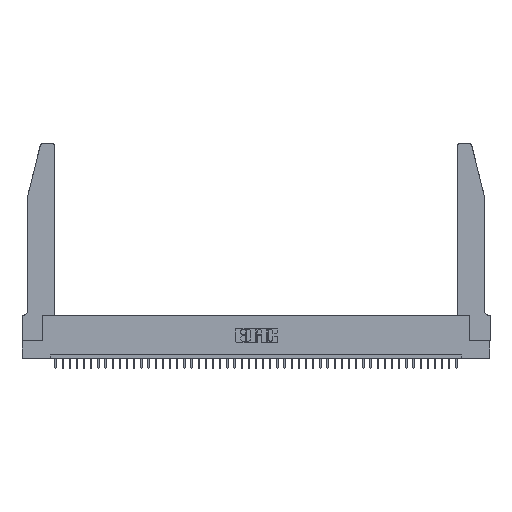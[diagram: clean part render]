
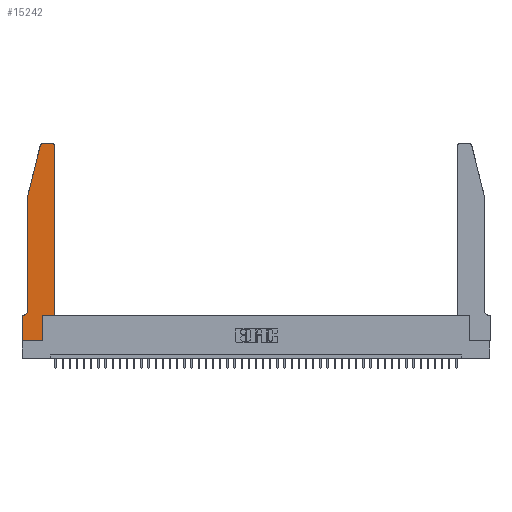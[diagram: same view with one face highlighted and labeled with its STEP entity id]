
A CAD part, top view. The second image highlights one B-rep face of the part: STEP entity #15242.
In plain terms, the highlighted planar face has unit normal (0, 0, 1).
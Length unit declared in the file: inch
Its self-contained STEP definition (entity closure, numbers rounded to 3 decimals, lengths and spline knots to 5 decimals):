
#481 = CARTESIAN_POINT ( 'NONE',  ( 0.25487, 2.72718, 0.37 ) ) ;
#940 = CIRCLE ( 'NONE', #44548, 0.07 ) ;
#1008 = CARTESIAN_POINT ( 'NONE',  ( 0.284, 2.75, 0.37 ) ) ;
#1127 = EDGE_CURVE ( 'NONE', #18805, #17591, #18720, .T. ) ;
#1324 = LINE ( 'NONE', #43206, #7119 ) ;
#1342 = EDGE_CURVE ( 'NONE', #5305, #18805, #2103, .T. ) ;
#2103 = CIRCLE ( 'NONE', #27911, 0.03 ) ;
#2881 = EDGE_CURVE ( 'NONE', #17591, #26068, #1324, .T. ) ;
#3198 = EDGE_CURVE ( 'NONE', #40577, #6330, #34597, .T. ) ;
#3223 = CARTESIAN_POINT ( 'NONE',  ( 0.2865, 0.35, 0.37 ) ) ;
#4160 = CARTESIAN_POINT ( 'NONE',  ( 0.4205, 2.75, 0.37 ) ) ;
#4233 = ORIENTED_EDGE ( 'NONE', *, *, #3198, .T. ) ;
#5054 = DIRECTION ( 'NONE',  ( -1., 0., 0. ) ) ;
#5305 = VERTEX_POINT ( 'NONE', #1008 ) ;
#6330 = VERTEX_POINT ( 'NONE', #33728 ) ;
#6615 = EDGE_CURVE ( 'NONE', #6330, #26174, #14759, .T. ) ;
#6768 = VECTOR ( 'NONE', #5054, 39.37008 ) ;
#7119 = VECTOR ( 'NONE', #15648, 39.37008 ) ;
#7630 = VERTEX_POINT ( 'NONE', #42210 ) ;
#9138 = DIRECTION ( 'NONE',  ( 1., 0., 0. ) ) ;
#9432 = VECTOR ( 'NONE', #25645, 39.37008 ) ;
#9655 = CARTESIAN_POINT ( 'NONE',  ( 0., 0., 0.37 ) ) ;
#10636 = ORIENTED_EDGE ( 'NONE', *, *, #41567, .T. ) ;
#11251 = ORIENTED_EDGE ( 'NONE', *, *, #2881, .T. ) ;
#11930 = DIRECTION ( 'NONE',  ( 0., 0., 1. ) ) ;
#12247 = CARTESIAN_POINT ( 'NONE',  ( 0.0755, 2., 0.37 ) ) ;
#12409 = DIRECTION ( 'NONE',  ( -1., 0., 0. ) ) ;
#12894 = DIRECTION ( 'NONE',  ( 1., 0., 0. ) ) ;
#14079 = CARTESIAN_POINT ( 'NONE',  ( 0., 0.35, 0.37 ) ) ;
#14759 = CIRCLE ( 'NONE', #40643, 0.03 ) ;
#15242 = ADVANCED_FACE ( 'NONE', ( #29955 ), #44088, .T. ) ;
#15648 = DIRECTION ( 'NONE',  ( 0., -1., 0. ) ) ;
#17333 = LINE ( 'NONE', #31433, #22160 ) ;
#17591 = VERTEX_POINT ( 'NONE', #12247 ) ;
#17934 = CARTESIAN_POINT ( 'NONE',  ( 0.4505, 0.35, 0.37 ) ) ;
#18720 = LINE ( 'NONE', #42195, #9432 ) ;
#18805 = VERTEX_POINT ( 'NONE', #481 ) ;
#18978 = CARTESIAN_POINT ( 'NONE',  ( 0.0055, 0.42, 0.37 ) ) ;
#19417 = ORIENTED_EDGE ( 'NONE', *, *, #25958, .T. ) ;
#19795 = VECTOR ( 'NONE', #28095, 39.37008 ) ;
#20864 = EDGE_CURVE ( 'NONE', #36734, #40577, #42946, .T. ) ;
#21230 = CARTESIAN_POINT ( 'NONE',  ( 0., 0., 0.37 ) ) ;
#21503 = ORIENTED_EDGE ( 'NONE', *, *, #20864, .T. ) ;
#22126 = DIRECTION ( 'NONE',  ( 1., 0., 0. ) ) ;
#22160 = VECTOR ( 'NONE', #38630, 39.37008 ) ;
#22268 = EDGE_CURVE ( 'NONE', #38720, #7630, #30485, .T. ) ;
#23160 = EDGE_LOOP ( 'NONE', ( #39592, #43818, #37624, #11251, #27389, #37796, #19417, #27024, #10636, #21503, #4233, #41970 ) ) ;
#23168 = CARTESIAN_POINT ( 'NONE',  ( 0., 0., 0.37 ) ) ;
#23807 = EDGE_CURVE ( 'NONE', #26174, #5305, #40235, .T. ) ;
#24648 = EDGE_CURVE ( 'NONE', #26068, #25562, #940, .T. ) ;
#25562 = VERTEX_POINT ( 'NONE', #34333 ) ;
#25645 = DIRECTION ( 'NONE',  ( -0.239, -0.971, 0. ) ) ;
#25958 = EDGE_CURVE ( 'NONE', #28944, #38720, #41449, .T. ) ;
#26068 = VERTEX_POINT ( 'NONE', #34950 ) ;
#26073 = DIRECTION ( 'NONE',  ( 0., 0., 1. ) ) ;
#26174 = VERTEX_POINT ( 'NONE', #4160 ) ;
#26617 = DIRECTION ( 'NONE',  ( 0., 0., -1. ) ) ;
#27024 = ORIENTED_EDGE ( 'NONE', *, *, #22268, .T. ) ;
#27389 = ORIENTED_EDGE ( 'NONE', *, *, #24648, .T. ) ;
#27911 = AXIS2_PLACEMENT_3D ( 'NONE', #28146, #38590, #45326 ) ;
#28095 = DIRECTION ( 'NONE',  ( 0., 1., 0. ) ) ;
#28146 = CARTESIAN_POINT ( 'NONE',  ( 0.284, 2.72, 0.37 ) ) ;
#28944 = VERTEX_POINT ( 'NONE', #14079 ) ;
#29955 = FACE_OUTER_BOUND ( 'NONE', #23160, .T. ) ;
#30485 = LINE ( 'NONE', #9655, #32506 ) ;
#31433 = CARTESIAN_POINT ( 'NONE',  ( 0.2865, 0.35, 0.37 ) ) ;
#32506 = VECTOR ( 'NONE', #12894, 39.37008 ) ;
#33234 = CARTESIAN_POINT ( 'NONE',  ( 0.0755, 0.35, 0.37 ) ) ;
#33728 = CARTESIAN_POINT ( 'NONE',  ( 0.4505, 2.72, 0.37 ) ) ;
#33906 = CARTESIAN_POINT ( 'NONE',  ( 0.4505, 0.35, 0.37 ) ) ;
#34333 = CARTESIAN_POINT ( 'NONE',  ( 0.0055, 0.35, 0.37 ) ) ;
#34597 = LINE ( 'NONE', #17934, #19795 ) ;
#34950 = CARTESIAN_POINT ( 'NONE',  ( 0.0755, 0.42, 0.37 ) ) ;
#35726 = VECTOR ( 'NONE', #37498, 39.37008 ) ;
#35764 = CARTESIAN_POINT ( 'NONE',  ( 0.4505, 0.35, 0.37 ) ) ;
#36696 = CARTESIAN_POINT ( 'NONE',  ( 0.4205, 2.72, 0.37 ) ) ;
#36723 = CARTESIAN_POINT ( 'NONE',  ( 0.2605, 2.75, 0.37 ) ) ;
#36734 = VERTEX_POINT ( 'NONE', #3223 ) ;
#37009 = EDGE_CURVE ( 'NONE', #25562, #28944, #44360, .T. ) ;
#37498 = DIRECTION ( 'NONE',  ( 0., -1., 0. ) ) ;
#37624 = ORIENTED_EDGE ( 'NONE', *, *, #1127, .T. ) ;
#37796 = ORIENTED_EDGE ( 'NONE', *, *, #37009, .T. ) ;
#38590 = DIRECTION ( 'NONE',  ( 0., 0., 1. ) ) ;
#38630 = DIRECTION ( 'NONE',  ( 0., 1., 0. ) ) ;
#38720 = VERTEX_POINT ( 'NONE', #21230 ) ;
#39592 = ORIENTED_EDGE ( 'NONE', *, *, #23807, .T. ) ;
#39718 = AXIS2_PLACEMENT_3D ( 'NONE', #40851, #11930, #9138 ) ;
#40235 = LINE ( 'NONE', #36723, #6768 ) ;
#40577 = VERTEX_POINT ( 'NONE', #33906 ) ;
#40643 = AXIS2_PLACEMENT_3D ( 'NONE', #36696, #26073, #22126 ) ;
#40667 = VECTOR ( 'NONE', #42710, 39.37008 ) ;
#40851 = CARTESIAN_POINT ( 'NONE',  ( 0., 0.35, 0.37 ) ) ;
#41449 = LINE ( 'NONE', #23168, #35726 ) ;
#41567 = EDGE_CURVE ( 'NONE', #7630, #36734, #17333, .T. ) ;
#41970 = ORIENTED_EDGE ( 'NONE', *, *, #6615, .T. ) ;
#42195 = CARTESIAN_POINT ( 'NONE',  ( 0.0755, 2., 0.37 ) ) ;
#42210 = CARTESIAN_POINT ( 'NONE',  ( 0.2865, 0., 0.37 ) ) ;
#42710 = DIRECTION ( 'NONE',  ( 1., 0., 0. ) ) ;
#42946 = LINE ( 'NONE', #35764, #40667 ) ;
#43206 = CARTESIAN_POINT ( 'NONE',  ( 0.0755, 2., 0.37 ) ) ;
#43782 = DIRECTION ( 'NONE',  ( -1., 0., 0. ) ) ;
#43818 = ORIENTED_EDGE ( 'NONE', *, *, #1342, .T. ) ;
#44088 = PLANE ( 'NONE',  #39718 ) ;
#44360 = LINE ( 'NONE', #33234, #45126 ) ;
#44548 = AXIS2_PLACEMENT_3D ( 'NONE', #18978, #26617, #43782 ) ;
#45126 = VECTOR ( 'NONE', #12409, 39.37008 ) ;
#45326 = DIRECTION ( 'NONE',  ( 1., 0., 0. ) ) ;
